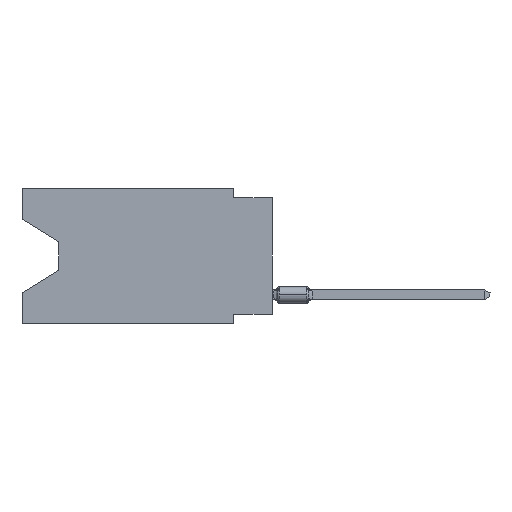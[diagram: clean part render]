
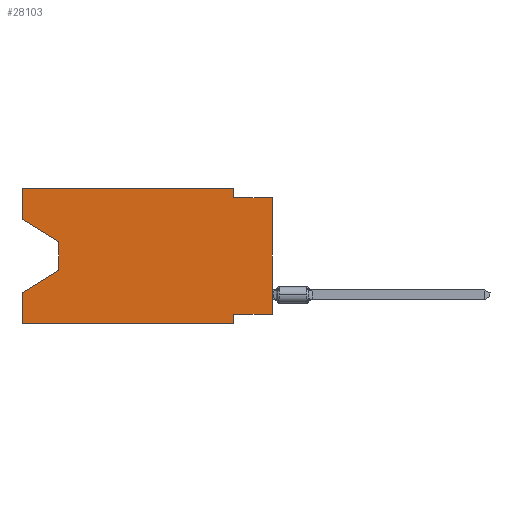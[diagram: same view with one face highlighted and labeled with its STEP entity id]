
A CAD part, left-side view. The second image highlights one B-rep face of the part: STEP entity #28103.
In plain terms, the highlighted planar face has unit normal (-1, 0, 0).
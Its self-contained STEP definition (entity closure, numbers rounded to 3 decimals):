
#346 = CARTESIAN_POINT ( 'NONE',  ( 0., 2.54, -8.89 ) ) ;
#956 = VERTEX_POINT ( 'NONE', #5274 ) ;
#1265 = CARTESIAN_POINT ( 'NONE',  ( 0., 0., 0. ) ) ;
#1281 = VECTOR ( 'NONE', #26246, 1000. ) ;
#1599 = VERTEX_POINT ( 'NONE', #27243 ) ;
#2242 = VECTOR ( 'NONE', #5453, 1000. ) ;
#3096 = LINE ( 'NONE', #14668, #1281 ) ;
#3309 = LINE ( 'NONE', #31992, #31577 ) ;
#3376 = CARTESIAN_POINT ( 'NONE',  ( 0., 16.383, 0. ) ) ;
#3877 = ORIENTED_EDGE ( 'NONE', *, *, #17515, .F. ) ;
#4396 = DIRECTION ( 'NONE',  ( 0., 0., -1. ) ) ;
#4471 = ORIENTED_EDGE ( 'NONE', *, *, #13585, .F. ) ;
#4551 = EDGE_CURVE ( 'NONE', #31732, #16134, #9246, .T. ) ;
#4750 = CARTESIAN_POINT ( 'NONE',  ( 0., 16.383, 0. ) ) ;
#5129 = VERTEX_POINT ( 'NONE', #27656 ) ;
#5267 = LINE ( 'NONE', #10966, #2242 ) ;
#5274 = CARTESIAN_POINT ( 'NONE',  ( 0., 16.383, 0. ) ) ;
#5453 = DIRECTION ( 'NONE',  ( 0., 0., -1. ) ) ;
#5731 = VECTOR ( 'NONE', #15223, 1000. ) ;
#6240 = EDGE_CURVE ( 'NONE', #28655, #12246, #25422, .T. ) ;
#7486 = VECTOR ( 'NONE', #4396, 1000. ) ;
#8421 = VECTOR ( 'NONE', #8682, 1000. ) ;
#8682 = DIRECTION ( 'NONE',  ( 0., -1., 0. ) ) ;
#9246 = LINE ( 'NONE', #346, #14402 ) ;
#9711 = LINE ( 'NONE', #21292, #19543 ) ;
#10435 = EDGE_CURVE ( 'NONE', #1599, #28655, #5267, .T. ) ;
#10966 = CARTESIAN_POINT ( 'NONE',  ( 0., 2.54, 0. ) ) ;
#11042 = CARTESIAN_POINT ( 'NONE',  ( 0., 2.54, -8.89 ) ) ;
#11621 = CARTESIAN_POINT ( 'NONE',  ( 0., 0., -8.255 ) ) ;
#11718 = CARTESIAN_POINT ( 'NONE',  ( 0., 2.54, -0.635 ) ) ;
#12129 = EDGE_CURVE ( 'NONE', #5129, #29573, #32280, .T. ) ;
#12246 = VERTEX_POINT ( 'NONE', #35527 ) ;
#12897 = EDGE_CURVE ( 'NONE', #25734, #12246, #15508, .T. ) ;
#13233 = CARTESIAN_POINT ( 'NONE',  ( 0., 16.383, -6.852 ) ) ;
#13297 = FACE_OUTER_BOUND ( 'NONE', #21472, .T. ) ;
#13585 = EDGE_CURVE ( 'NONE', #956, #1599, #3096, .T. ) ;
#13672 = DIRECTION ( 'NONE',  ( 1., 0., 0. ) ) ;
#14357 = VERTEX_POINT ( 'NONE', #13233 ) ;
#14402 = VECTOR ( 'NONE', #20465, 1000. ) ;
#14457 = ORIENTED_EDGE ( 'NONE', *, *, #25131, .T. ) ;
#14668 = CARTESIAN_POINT ( 'NONE',  ( 0., 16.383, 0. ) ) ;
#14950 = DIRECTION ( 'NONE',  ( 0., 0., 1. ) ) ;
#15223 = DIRECTION ( 'NONE',  ( 0., 1., 0. ) ) ;
#15508 = LINE ( 'NONE', #1265, #22084 ) ;
#15878 = ORIENTED_EDGE ( 'NONE', *, *, #23093, .T. ) ;
#16134 = VERTEX_POINT ( 'NONE', #11042 ) ;
#16340 = DIRECTION ( 'NONE',  ( 0., 0., -1. ) ) ;
#17513 = LINE ( 'NONE', #11621, #5731 ) ;
#17515 = EDGE_CURVE ( 'NONE', #25734, #31732, #17513, .T. ) ;
#18095 = CARTESIAN_POINT ( 'NONE',  ( 0., 2.54, -8.255 ) ) ;
#19543 = VECTOR ( 'NONE', #27371, 1000. ) ;
#19835 = ORIENTED_EDGE ( 'NONE', *, *, #35875, .F. ) ;
#20465 = DIRECTION ( 'NONE',  ( 0., 0., -1. ) ) ;
#20858 = CARTESIAN_POINT ( 'NONE',  ( 0., 16.383, -2.038 ) ) ;
#21292 = CARTESIAN_POINT ( 'NONE',  ( 0., 16.383, -8.89 ) ) ;
#21472 = EDGE_LOOP ( 'NONE', ( #33683, #15878, #14457, #32352, #36631, #25040, #3877, #27206, #35820, #24607, #4471, #19835 ) ) ;
#21716 = DIRECTION ( 'NONE',  ( 0., 0.855, -0.519 ) ) ;
#22084 = VECTOR ( 'NONE', #27447, 1000. ) ;
#23093 = EDGE_CURVE ( 'NONE', #29573, #34519, #30986, .T. ) ;
#24607 = ORIENTED_EDGE ( 'NONE', *, *, #10435, .F. ) ;
#25040 = ORIENTED_EDGE ( 'NONE', *, *, #4551, .F. ) ;
#25131 = EDGE_CURVE ( 'NONE', #34519, #14357, #33682, .T. ) ;
#25362 = VERTEX_POINT ( 'NONE', #33174 ) ;
#25422 = LINE ( 'NONE', #34745, #8421 ) ;
#25734 = VERTEX_POINT ( 'NONE', #34489 ) ;
#26246 = DIRECTION ( 'NONE',  ( 0., -1., 0. ) ) ;
#26748 = EDGE_CURVE ( 'NONE', #25362, #14357, #29379, .T. ) ;
#27206 = ORIENTED_EDGE ( 'NONE', *, *, #12897, .T. ) ;
#27243 = CARTESIAN_POINT ( 'NONE',  ( 0., 2.54, 0. ) ) ;
#27371 = DIRECTION ( 'NONE',  ( 0., -1., 0. ) ) ;
#27447 = DIRECTION ( 'NONE',  ( 0., 0., 1. ) ) ;
#27656 = CARTESIAN_POINT ( 'NONE',  ( 0., 16.383, -2.038 ) ) ;
#28045 = EDGE_CURVE ( 'NONE', #25362, #16134, #9711, .T. ) ;
#28103 = ADVANCED_FACE ( 'NONE', ( #13297 ), #33620, .F. ) ;
#28655 = VERTEX_POINT ( 'NONE', #11718 ) ;
#29379 = LINE ( 'NONE', #3376, #36229 ) ;
#29573 = VERTEX_POINT ( 'NONE', #31489 ) ;
#30054 = VECTOR ( 'NONE', #21716, 1000. ) ;
#30986 = LINE ( 'NONE', #31175, #7486 ) ;
#31175 = CARTESIAN_POINT ( 'NONE',  ( 0., 13.97, -3.505 ) ) ;
#31489 = CARTESIAN_POINT ( 'NONE',  ( 0., 13.97, -3.505 ) ) ;
#31577 = VECTOR ( 'NONE', #35049, 1000. ) ;
#31732 = VERTEX_POINT ( 'NONE', #18095 ) ;
#31992 = CARTESIAN_POINT ( 'NONE',  ( 0., 16.383, 0. ) ) ;
#32280 = LINE ( 'NONE', #20858, #37280 ) ;
#32352 = ORIENTED_EDGE ( 'NONE', *, *, #26748, .F. ) ;
#33174 = CARTESIAN_POINT ( 'NONE',  ( 0., 16.383, -8.89 ) ) ;
#33513 = AXIS2_PLACEMENT_3D ( 'NONE', #4750, #13672, #16340 ) ;
#33620 = PLANE ( 'NONE',  #33513 ) ;
#33682 = LINE ( 'NONE', #36003, #30054 ) ;
#33683 = ORIENTED_EDGE ( 'NONE', *, *, #12129, .T. ) ;
#34234 = CARTESIAN_POINT ( 'NONE',  ( 0., 13.97, -5.385 ) ) ;
#34489 = CARTESIAN_POINT ( 'NONE',  ( 0., 0., -8.255 ) ) ;
#34519 = VERTEX_POINT ( 'NONE', #34234 ) ;
#34585 = DIRECTION ( 'NONE',  ( 0., -0.855, -0.519 ) ) ;
#34745 = CARTESIAN_POINT ( 'NONE',  ( 0., 0., -0.635 ) ) ;
#35049 = DIRECTION ( 'NONE',  ( 0., 0., 1. ) ) ;
#35527 = CARTESIAN_POINT ( 'NONE',  ( 0., 0., -0.635 ) ) ;
#35820 = ORIENTED_EDGE ( 'NONE', *, *, #6240, .F. ) ;
#35875 = EDGE_CURVE ( 'NONE', #5129, #956, #3309, .T. ) ;
#36003 = CARTESIAN_POINT ( 'NONE',  ( 0., 13.97, -5.385 ) ) ;
#36229 = VECTOR ( 'NONE', #14950, 1000. ) ;
#36631 = ORIENTED_EDGE ( 'NONE', *, *, #28045, .T. ) ;
#37280 = VECTOR ( 'NONE', #34585, 1000. ) ;
